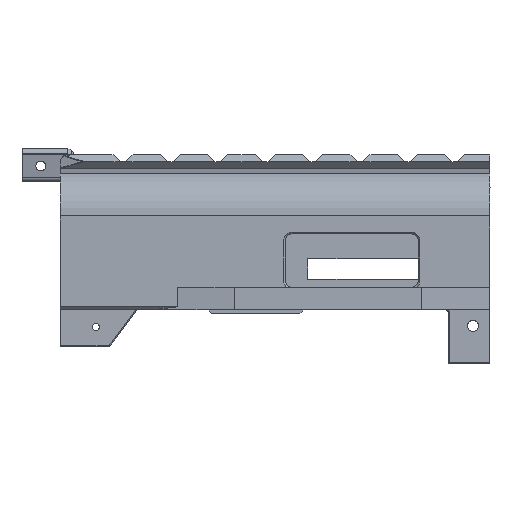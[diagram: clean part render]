
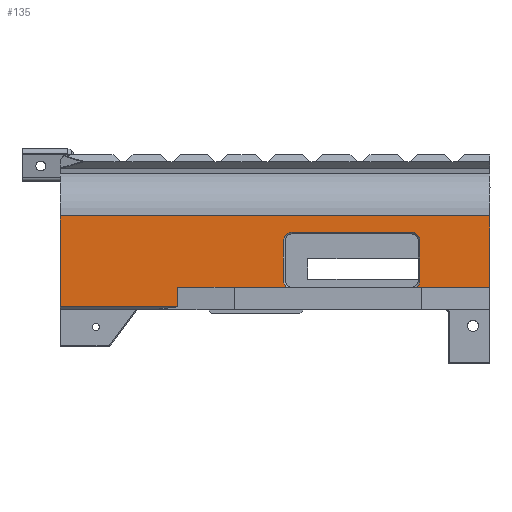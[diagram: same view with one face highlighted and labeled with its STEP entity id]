
A CAD part, top view. The second image highlights one B-rep face of the part: STEP entity #135.
In plain terms, the highlighted planar face has unit normal (0, 0, 1).
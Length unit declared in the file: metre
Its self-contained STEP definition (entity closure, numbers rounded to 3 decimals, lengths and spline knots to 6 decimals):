
#135=ADVANCED_FACE('0:686',(#504),#505,.T.);
#504=FACE_OUTER_BOUND('',#1105,.T.);
#505=PLANE('',#1106);
#1105=EDGE_LOOP('',(#2301,#2302,#2303,#2304,#2305,#2306,#2307,#2308,#2309,#2310,#2311,#2312,#2313,#2314));
#1106=AXIS2_PLACEMENT_3D('',#2315,#2316,#2317);
#2301=ORIENTED_EDGE('',*,*,#4147,.F.);
#2302=ORIENTED_EDGE('',*,*,#4278,.F.);
#2303=ORIENTED_EDGE('',*,*,#4245,.F.);
#2304=ORIENTED_EDGE('',*,*,#4279,.T.);
#2305=ORIENTED_EDGE('',*,*,#4280,.T.);
#2306=ORIENTED_EDGE('',*,*,#4281,.T.);
#2307=ORIENTED_EDGE('',*,*,#4153,.F.);
#2308=ORIENTED_EDGE('',*,*,#4282,.T.);
#2309=ORIENTED_EDGE('',*,*,#4283,.T.);
#2310=ORIENTED_EDGE('',*,*,#4284,.T.);
#2311=ORIENTED_EDGE('',*,*,#4285,.T.);
#2312=ORIENTED_EDGE('',*,*,#4286,.T.);
#2313=ORIENTED_EDGE('',*,*,#4287,.T.);
#2314=ORIENTED_EDGE('',*,*,#4288,.T.);
#2315=CARTESIAN_POINT('',(-0.020072,0.047361,0.0211));
#2316=DIRECTION('',(0.,0.,1.0));
#2317=DIRECTION('',(1.0,0.0,0.));
#4147=EDGE_CURVE('0:2927',#5118,#5119,#5120,.T.);
#4153=EDGE_CURVE('0:2930',#5129,#5131,#5132,.T.);
#4245=EDGE_CURVE('0:2933',#5295,#5293,#5297,.T.);
#4278=EDGE_CURVE('0:2936',#5293,#5118,#5360,.T.);
#4279=EDGE_CURVE('0:1364',#5295,#5361,#5362,.T.);
#4280=EDGE_CURVE('0:1499',#5361,#5363,#5364,.T.);
#4281=EDGE_CURVE('0:1661',#5363,#5131,#5365,.T.);
#4282=EDGE_CURVE('0:2771',#5129,#5366,#5367,.T.);
#4283=EDGE_CURVE('0:2285',#5366,#5368,#5369,.T.);
#4284=EDGE_CURVE('0:2765',#5368,#5370,#5371,.T.);
#4285=EDGE_CURVE('0:1487',#5370,#5372,#5373,.T.);
#4286=EDGE_CURVE('0:2762',#5372,#5374,#5375,.T.);
#4287=EDGE_CURVE('0:2276',#5374,#5376,#5377,.T.);
#4288=EDGE_CURVE('0:2774',#5376,#5119,#5378,.T.);
#5118=VERTEX_POINT('',#6676);
#5119=VERTEX_POINT('',#6677);
#5120=LINE('',#6678,#6679);
#5129=VERTEX_POINT('',#6701);
#5131=VERTEX_POINT('',#6712);
#5132=LINE('',#6713,#6714);
#5293=VERTEX_POINT('',#6959);
#5295=VERTEX_POINT('',#6961);
#5297=LINE('',#6963,#6964);
#5360=LINE('',#7059,#7060);
#5361=VERTEX_POINT('',#7061);
#5362=LINE('',#7062,#7063);
#5363=VERTEX_POINT('',#7064);
#5364=LINE('',#7065,#7066);
#5365=LINE('',#7067,#7068);
#5366=VERTEX_POINT('',#7069);
#5367=CIRCLE('',#7070,0.0038);
#5368=VERTEX_POINT('',#7071);
#5369=LINE('',#7072,#7073);
#5370=VERTEX_POINT('',#7074);
#5371=CIRCLE('',#7075,0.0038);
#5372=VERTEX_POINT('',#7076);
#5373=LINE('',#7077,#7078);
#5374=VERTEX_POINT('',#7079);
#5375=CIRCLE('',#7080,0.0038);
#5376=VERTEX_POINT('',#7081);
#5377=LINE('',#7082,#7083);
#5378=CIRCLE('',#7084,0.0038);
#6676=CARTESIAN_POINT('',(0.011678,0.015811,0.0211));
#6677=CARTESIAN_POINT('',(-0.020846,0.015811,0.0211));
#6678=CARTESIAN_POINT('',(-0.106587,0.015811,0.0211));
#6679=VECTOR('',#8320,1.0);
#6701=CARTESIAN_POINT('',(-0.078355,0.015811,0.0211));
#6712=CARTESIAN_POINT('',(-0.126814,0.015811,0.0211));
#6713=CARTESIAN_POINT('',(-0.106587,0.015811,0.0211));
#6714=VECTOR('',#8324,1.0);
#6959=CARTESIAN_POINT('',(0.011678,0.047361,0.0211));
#6961=CARTESIAN_POINT('',(-0.178704,0.047361,0.0211));
#6963=CARTESIAN_POINT('',(-0.020072,0.047361,0.0211));
#6964=VECTOR('',#8436,1.0);
#7059=CARTESIAN_POINT('',(0.011678,0.047361,0.0211));
#7060=VECTOR('',#8469,1.0);
#7061=CARTESIAN_POINT('',(-0.178704,0.007104,0.0211));
#7062=CARTESIAN_POINT('',(-0.178704,0.030072,0.0211));
#7063=VECTOR('',#8470,1.0);
#7064=CARTESIAN_POINT('',(-0.126814,0.007104,0.0211));
#7065=CARTESIAN_POINT('',(-0.089922,0.007104,0.0211));
#7066=VECTOR('',#8471,1.0);
#7067=CARTESIAN_POINT('',(-0.126814,0.047361,0.0211));
#7068=VECTOR('',#8472,1.0);
#7069=CARTESIAN_POINT('',(-0.079822,0.018811,0.0211));
#7070=AXIS2_PLACEMENT_3D('',#8473,#8474,#8475);
#7071=CARTESIAN_POINT('',(-0.079822,0.036397,0.0211));
#7072=CARTESIAN_POINT('',(-0.079822,0.047361,0.0211));
#7073=VECTOR('',#8476,1.0);
#7074=CARTESIAN_POINT('',(-0.076022,0.040197,0.0211));
#7075=AXIS2_PLACEMENT_3D('',#8477,#8478,#8479);
#7076=CARTESIAN_POINT('',(-0.023178,0.040197,0.0211));
#7077=CARTESIAN_POINT('',(-0.020072,0.040197,0.0211));
#7078=VECTOR('',#8480,1.0);
#7079=CARTESIAN_POINT('',(-0.019378,0.036397,0.0211));
#7080=AXIS2_PLACEMENT_3D('',#8481,#8482,#8483);
#7081=CARTESIAN_POINT('',(-0.019378,0.018811,0.0211));
#7082=CARTESIAN_POINT('',(-0.019378,0.047361,0.0211));
#7083=VECTOR('',#8484,1.0);
#7084=AXIS2_PLACEMENT_3D('',#8485,#8486,#8487);
#8320=DIRECTION('',(-1.0,0.,0.));
#8324=DIRECTION('',(-1.0,0.,0.));
#8436=DIRECTION('',(1.0,0.0,0.));
#8469=DIRECTION('',(0.,-1.0,0.));
#8470=DIRECTION('',(0.0,-1.0,-0.0));
#8471=DIRECTION('',(1.0,0.,0.));
#8472=DIRECTION('',(0.,1.0,0.));
#8473=CARTESIAN_POINT('',(-0.076022,0.018811,0.0211));
#8474=DIRECTION('',(0.,0.,-1.0));
#8475=DIRECTION('',(1.0,0.,0.));
#8476=DIRECTION('',(0.,1.0,0.));
#8477=CARTESIAN_POINT('',(-0.076022,0.036397,0.0211));
#8478=DIRECTION('',(0.,0.,-1.0));
#8479=DIRECTION('',(1.0,0.,0.));
#8480=DIRECTION('',(1.0,0.0,0.));
#8481=CARTESIAN_POINT('',(-0.023178,0.036397,0.0211));
#8482=DIRECTION('',(0.,0.,-1.0));
#8483=DIRECTION('',(1.0,0.,0.));
#8484=DIRECTION('',(0.,-1.0,0.));
#8485=CARTESIAN_POINT('',(-0.023178,0.018811,0.0211));
#8486=DIRECTION('',(0.,0.,-1.0));
#8487=DIRECTION('',(1.0,0.,0.));
